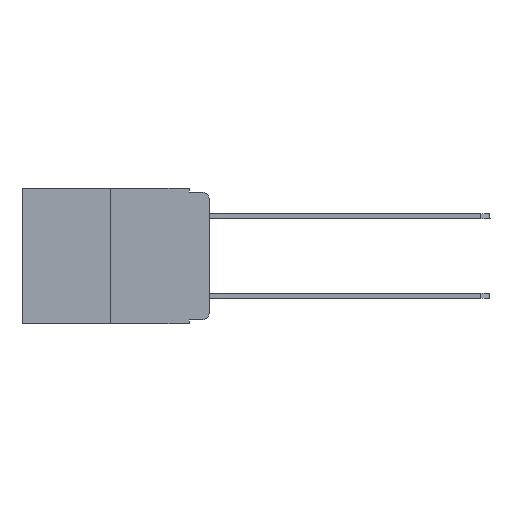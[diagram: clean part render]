
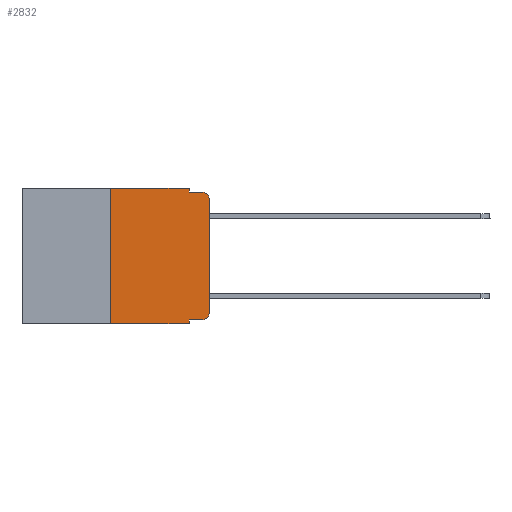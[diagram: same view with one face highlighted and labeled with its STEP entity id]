
A CAD part, left-side view. The second image highlights one B-rep face of the part: STEP entity #2832.
In plain terms, the highlighted planar face has unit normal (-1, 0, 0).
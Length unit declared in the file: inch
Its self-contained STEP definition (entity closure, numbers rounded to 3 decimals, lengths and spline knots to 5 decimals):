
#685 = ORIENTED_EDGE ( 'NONE', *, *, #19682, .T. ) ;
#747 = EDGE_CURVE ( 'NONE', #6896, #19790, #4857, .T. ) ;
#854 = VECTOR ( 'NONE', #11563, 39.37008 ) ;
#874 = VECTOR ( 'NONE', #14836, 39.37008 ) ;
#1215 = CIRCLE ( 'NONE', #16502, 0.02 ) ;
#1979 = ORIENTED_EDGE ( 'NONE', *, *, #4500, .F. ) ;
#2553 = ORIENTED_EDGE ( 'NONE', *, *, #7949, .T. ) ;
#2622 = AXIS2_PLACEMENT_3D ( 'NONE', #11985, #4965, #3295 ) ;
#2832 = ADVANCED_FACE ( 'NONE', ( #12213 ), #3742, .F. ) ;
#2935 = LINE ( 'NONE', #14961, #8693 ) ;
#2974 = LINE ( 'NONE', #4759, #854 ) ;
#3295 = DIRECTION ( 'NONE',  ( 0., 0., -1. ) ) ;
#3560 = VERTEX_POINT ( 'NONE', #17842 ) ;
#3604 = CIRCLE ( 'NONE', #11103, 0.02 ) ;
#3742 = PLANE ( 'NONE',  #2622 ) ;
#3857 = DIRECTION ( 'NONE',  ( -1., 0., 0. ) ) ;
#4025 = DIRECTION ( 'NONE',  ( 0., -1., 0. ) ) ;
#4321 = VERTEX_POINT ( 'NONE', #9341 ) ;
#4460 = CARTESIAN_POINT ( 'NONE',  ( 0., 0.473, 0. ) ) ;
#4500 = EDGE_CURVE ( 'NONE', #6896, #21391, #2974, .T. ) ;
#4660 = CARTESIAN_POINT ( 'NONE',  ( 0., 0.051, 0. ) ) ;
#4759 = CARTESIAN_POINT ( 'NONE',  ( 0., 0.25, 0. ) ) ;
#4857 = LINE ( 'NONE', #8200, #10528 ) ;
#4965 = DIRECTION ( 'NONE',  ( 1., 0., 0. ) ) ;
#5203 = VERTEX_POINT ( 'NONE', #12281 ) ;
#6397 = DIRECTION ( 'NONE',  ( 0., -1., 0. ) ) ;
#6896 = VERTEX_POINT ( 'NONE', #7449 ) ;
#7311 = ORIENTED_EDGE ( 'NONE', *, *, #747, .T. ) ;
#7449 = CARTESIAN_POINT ( 'NONE',  ( 0., 0.25, -0.343 ) ) ;
#7600 = LINE ( 'NONE', #19532, #874 ) ;
#7649 = EDGE_CURVE ( 'NONE', #5203, #19790, #18223, .T. ) ;
#7949 = EDGE_CURVE ( 'NONE', #14244, #4321, #14962, .T. ) ;
#8143 = CARTESIAN_POINT ( 'NONE',  ( 0., 0.02, -0.03 ) ) ;
#8200 = CARTESIAN_POINT ( 'NONE',  ( 0., 0.473, -0.343 ) ) ;
#8283 = ORIENTED_EDGE ( 'NONE', *, *, #7649, .F. ) ;
#8691 = ORIENTED_EDGE ( 'NONE', *, *, #16997, .F. ) ;
#8693 = VECTOR ( 'NONE', #6397, 39.37008 ) ;
#8961 = CARTESIAN_POINT ( 'NONE',  ( 0., 0.25, 0. ) ) ;
#9341 = CARTESIAN_POINT ( 'NONE',  ( 0., 0., -0.03 ) ) ;
#9649 = DIRECTION ( 'NONE',  ( 0., 0., -1. ) ) ;
#9870 = CARTESIAN_POINT ( 'NONE',  ( 0., 0.051, 0. ) ) ;
#10432 = CARTESIAN_POINT ( 'NONE',  ( 0., 0.02, -0.313 ) ) ;
#10528 = VECTOR ( 'NONE', #15436, 39.37008 ) ;
#10648 = DIRECTION ( 'NONE',  ( 0., 0., -1. ) ) ;
#10794 = EDGE_CURVE ( 'NONE', #5203, #3560, #2935, .T. ) ;
#11070 = VERTEX_POINT ( 'NONE', #11679 ) ;
#11103 = AXIS2_PLACEMENT_3D ( 'NONE', #10432, #3857, #10648 ) ;
#11485 = VERTEX_POINT ( 'NONE', #20334 ) ;
#11563 = DIRECTION ( 'NONE',  ( 0., 0., 1. ) ) ;
#11679 = CARTESIAN_POINT ( 'NONE',  ( 0., 0.051, -0.01 ) ) ;
#11749 = VECTOR ( 'NONE', #14856, 39.37008 ) ;
#11911 = VECTOR ( 'NONE', #9649, 39.37008 ) ;
#11985 = CARTESIAN_POINT ( 'NONE',  ( 0., 0.473, 0. ) ) ;
#12213 = FACE_OUTER_BOUND ( 'NONE', #18346, .T. ) ;
#12281 = CARTESIAN_POINT ( 'NONE',  ( 0., 0.051, -0.333 ) ) ;
#12310 = EDGE_CURVE ( 'NONE', #11070, #11485, #7600, .T. ) ;
#12421 = EDGE_CURVE ( 'NONE', #4321, #11485, #1215, .T. ) ;
#12847 = VERTEX_POINT ( 'NONE', #4660 ) ;
#12949 = ORIENTED_EDGE ( 'NONE', *, *, #10794, .T. ) ;
#13881 = DIRECTION ( 'NONE',  ( 0., 0., -1. ) ) ;
#14106 = LINE ( 'NONE', #20988, #14185 ) ;
#14185 = VECTOR ( 'NONE', #13881, 39.37008 ) ;
#14244 = VERTEX_POINT ( 'NONE', #17116 ) ;
#14463 = ORIENTED_EDGE ( 'NONE', *, *, #12310, .F. ) ;
#14627 = EDGE_CURVE ( 'NONE', #12847, #11070, #14106, .T. ) ;
#14836 = DIRECTION ( 'NONE',  ( 0., -1., 0. ) ) ;
#14856 = DIRECTION ( 'NONE',  ( 0., 0., 1. ) ) ;
#14936 = DIRECTION ( 'NONE',  ( -1., 0., 0. ) ) ;
#14961 = CARTESIAN_POINT ( 'NONE',  ( 0., 0.051, -0.333 ) ) ;
#14962 = LINE ( 'NONE', #20202, #11749 ) ;
#15436 = DIRECTION ( 'NONE',  ( 0., -1., 0. ) ) ;
#16150 = LINE ( 'NONE', #4460, #21659 ) ;
#16211 = CARTESIAN_POINT ( 'NONE',  ( 0., 0.051, -0.343 ) ) ;
#16495 = DIRECTION ( 'NONE',  ( 0., 0., -1. ) ) ;
#16502 = AXIS2_PLACEMENT_3D ( 'NONE', #8143, #14936, #16495 ) ;
#16997 = EDGE_CURVE ( 'NONE', #21391, #12847, #16150, .T. ) ;
#17116 = CARTESIAN_POINT ( 'NONE',  ( 0., 0., -0.313 ) ) ;
#17370 = ORIENTED_EDGE ( 'NONE', *, *, #14627, .F. ) ;
#17842 = CARTESIAN_POINT ( 'NONE',  ( 0., 0.02, -0.333 ) ) ;
#18223 = LINE ( 'NONE', #9870, #11911 ) ;
#18346 = EDGE_LOOP ( 'NONE', ( #2553, #21965, #14463, #17370, #8691, #1979, #7311, #8283, #12949, #685 ) ) ;
#19532 = CARTESIAN_POINT ( 'NONE',  ( 0., 0.051, -0.01 ) ) ;
#19682 = EDGE_CURVE ( 'NONE', #3560, #14244, #3604, .T. ) ;
#19790 = VERTEX_POINT ( 'NONE', #16211 ) ;
#20202 = CARTESIAN_POINT ( 'NONE',  ( 0., 0., 0. ) ) ;
#20334 = CARTESIAN_POINT ( 'NONE',  ( 0., 0.02, -0.01 ) ) ;
#20988 = CARTESIAN_POINT ( 'NONE',  ( 0., 0.051, 0. ) ) ;
#21391 = VERTEX_POINT ( 'NONE', #8961 ) ;
#21659 = VECTOR ( 'NONE', #4025, 39.37008 ) ;
#21965 = ORIENTED_EDGE ( 'NONE', *, *, #12421, .T. ) ;
